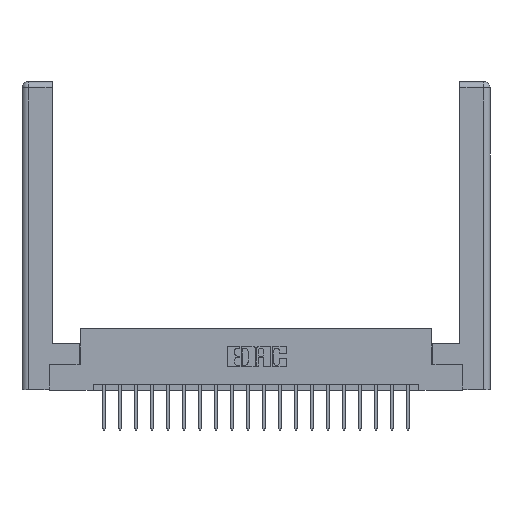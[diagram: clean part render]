
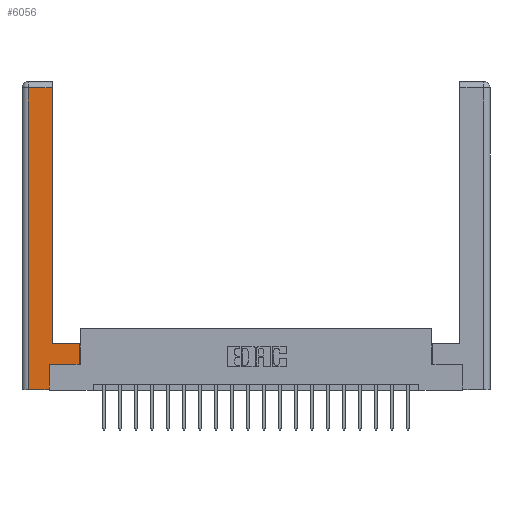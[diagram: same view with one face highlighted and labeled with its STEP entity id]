
A CAD part, top view. The second image highlights one B-rep face of the part: STEP entity #6056.
In plain terms, the highlighted planar face has unit normal (0, 0, 1).
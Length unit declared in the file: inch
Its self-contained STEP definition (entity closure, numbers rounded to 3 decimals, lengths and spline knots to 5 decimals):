
#234 = CARTESIAN_POINT ( 'NONE',  ( 0.265, 0.245, 0. ) ) ;
#335 = ORIENTED_EDGE ( 'NONE', *, *, #2428, .T. ) ;
#445 = CARTESIAN_POINT ( 'NONE',  ( 0.0615, 0., 0. ) ) ;
#495 = LINE ( 'NONE', #1268, #7097 ) ;
#674 = VECTOR ( 'NONE', #3154, 39.37008 ) ;
#977 = LINE ( 'NONE', #6207, #17706 ) ;
#1192 = FACE_OUTER_BOUND ( 'NONE', #4812, .T. ) ;
#1229 = EDGE_CURVE ( 'NONE', #12842, #9808, #495, .T. ) ;
#1268 = CARTESIAN_POINT ( 'NONE',  ( 0.265, 0.245, 0. ) ) ;
#1581 = CARTESIAN_POINT ( 'NONE',  ( 0.0615, 2.94, 0. ) ) ;
#1654 = EDGE_CURVE ( 'NONE', #17828, #19054, #977, .T. ) ;
#2212 = EDGE_CURVE ( 'NONE', #3257, #5081, #4156, .T. ) ;
#2428 = EDGE_CURVE ( 'NONE', #8746, #17828, #12055, .T. ) ;
#2702 = CARTESIAN_POINT ( 'NONE',  ( 0.295, 0.45, 0. ) ) ;
#2964 = DIRECTION ( 'NONE',  ( 1., 0., 0. ) ) ;
#3154 = DIRECTION ( 'NONE',  ( 1., 0., 0. ) ) ;
#3257 = VERTEX_POINT ( 'NONE', #4371 ) ;
#3743 = VECTOR ( 'NONE', #5194, 39.37008 ) ;
#4156 = LINE ( 'NONE', #9016, #13034 ) ;
#4371 = CARTESIAN_POINT ( 'NONE',  ( 0.565, 0.245, 0. ) ) ;
#4666 = VECTOR ( 'NONE', #9494, 39.37008 ) ;
#4812 = EDGE_LOOP ( 'NONE', ( #17643, #335, #14201, #13804, #14871, #10285, #20224, #17281 ) ) ;
#5081 = VERTEX_POINT ( 'NONE', #10153 ) ;
#5194 = DIRECTION ( 'NONE',  ( 0., 1., 0. ) ) ;
#5295 = LINE ( 'NONE', #10890, #15182 ) ;
#5647 = DIRECTION ( 'NONE',  ( -1., 0., 0. ) ) ;
#5772 = CARTESIAN_POINT ( 'NONE',  ( 0.265, 0., 0. ) ) ;
#6004 = AXIS2_PLACEMENT_3D ( 'NONE', #10275, #11264, #5647 ) ;
#6056 = ADVANCED_FACE ( 'NONE', ( #1192 ), #6120, .F. ) ;
#6120 = PLANE ( 'NONE',  #6004 ) ;
#6207 = CARTESIAN_POINT ( 'NONE',  ( 0.0615, 0., 0. ) ) ;
#6360 = EDGE_CURVE ( 'NONE', #19054, #12842, #18159, .T. ) ;
#6533 = CARTESIAN_POINT ( 'NONE',  ( 0.295, 3., 0. ) ) ;
#7097 = VECTOR ( 'NONE', #17562, 39.37008 ) ;
#8746 = VERTEX_POINT ( 'NONE', #10026 ) ;
#8868 = EDGE_CURVE ( 'NONE', #18206, #8746, #18184, .T. ) ;
#9016 = CARTESIAN_POINT ( 'NONE',  ( 0.565, 0.45, 0. ) ) ;
#9494 = DIRECTION ( 'NONE',  ( -1., 0., 0. ) ) ;
#9579 = CARTESIAN_POINT ( 'NONE',  ( 0.265, 0., 0. ) ) ;
#9808 = VERTEX_POINT ( 'NONE', #234 ) ;
#10026 = CARTESIAN_POINT ( 'NONE',  ( 0.295, 2.94, 0. ) ) ;
#10050 = CARTESIAN_POINT ( 'NONE',  ( 0.295, 0.45, 0. ) ) ;
#10153 = CARTESIAN_POINT ( 'NONE',  ( 0.565, 0.45, 0. ) ) ;
#10275 = CARTESIAN_POINT ( 'NONE',  ( 0., 0., 0. ) ) ;
#10285 = ORIENTED_EDGE ( 'NONE', *, *, #14315, .T. ) ;
#10430 = DIRECTION ( 'NONE',  ( 0., 1., 0. ) ) ;
#10890 = CARTESIAN_POINT ( 'NONE',  ( 0.565, 0.245, 0. ) ) ;
#11264 = DIRECTION ( 'NONE',  ( 0., 0., -1. ) ) ;
#11317 = DIRECTION ( 'NONE',  ( 0., -1., 0. ) ) ;
#12055 = LINE ( 'NONE', #1581, #4666 ) ;
#12842 = VERTEX_POINT ( 'NONE', #5772 ) ;
#13034 = VECTOR ( 'NONE', #10430, 39.37008 ) ;
#13804 = ORIENTED_EDGE ( 'NONE', *, *, #6360, .T. ) ;
#13827 = VECTOR ( 'NONE', #16429, 39.37008 ) ;
#14201 = ORIENTED_EDGE ( 'NONE', *, *, #1654, .T. ) ;
#14315 = EDGE_CURVE ( 'NONE', #9808, #3257, #5295, .T. ) ;
#14871 = ORIENTED_EDGE ( 'NONE', *, *, #1229, .T. ) ;
#15182 = VECTOR ( 'NONE', #2964, 39.37008 ) ;
#15602 = LINE ( 'NONE', #10050, #13827 ) ;
#15772 = EDGE_CURVE ( 'NONE', #5081, #18206, #15602, .T. ) ;
#16429 = DIRECTION ( 'NONE',  ( -1., 0., 0. ) ) ;
#17281 = ORIENTED_EDGE ( 'NONE', *, *, #15772, .T. ) ;
#17562 = DIRECTION ( 'NONE',  ( 0., 1., 0. ) ) ;
#17643 = ORIENTED_EDGE ( 'NONE', *, *, #8868, .T. ) ;
#17706 = VECTOR ( 'NONE', #11317, 39.37008 ) ;
#17828 = VERTEX_POINT ( 'NONE', #18918 ) ;
#18159 = LINE ( 'NONE', #9579, #674 ) ;
#18184 = LINE ( 'NONE', #6533, #3743 ) ;
#18206 = VERTEX_POINT ( 'NONE', #2702 ) ;
#18918 = CARTESIAN_POINT ( 'NONE',  ( 0.0615, 2.94, 0. ) ) ;
#19054 = VERTEX_POINT ( 'NONE', #445 ) ;
#20224 = ORIENTED_EDGE ( 'NONE', *, *, #2212, .T. ) ;
